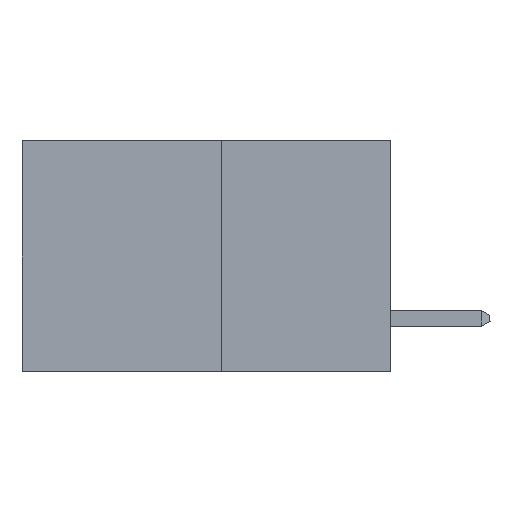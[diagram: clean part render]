
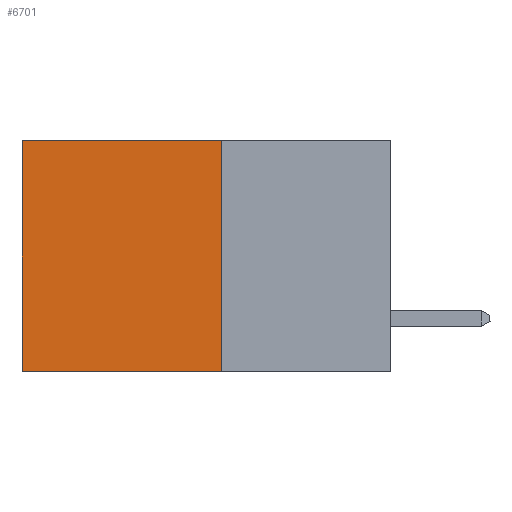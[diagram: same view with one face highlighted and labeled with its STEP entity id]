
A CAD part, left-side view. The second image highlights one B-rep face of the part: STEP entity #6701.
In plain terms, the highlighted planar face has unit normal (-1, 0, 0).
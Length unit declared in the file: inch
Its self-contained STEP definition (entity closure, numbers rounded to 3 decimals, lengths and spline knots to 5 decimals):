
#8 = LINE ( 'NONE', #911, #14515 ) ;
#165 = EDGE_CURVE ( 'NONE', #3886, #6773, #2893, .T. ) ;
#326 = EDGE_CURVE ( 'NONE', #501, #8217, #6914, .T. ) ;
#501 = VERTEX_POINT ( 'NONE', #16231 ) ;
#911 = CARTESIAN_POINT ( 'NONE',  ( 0.277, 0.27, -0.37 ) ) ;
#1520 = DIRECTION ( 'NONE',  ( 1., 0., 0. ) ) ;
#1638 = DIRECTION ( 'NONE',  ( 0., 0., -1. ) ) ;
#2648 = VECTOR ( 'NONE', #5452, 39.37008 ) ;
#2655 = VECTOR ( 'NONE', #4119, 39.37008 ) ;
#2671 = CARTESIAN_POINT ( 'NONE',  ( 0.277, 0.27, -0.37 ) ) ;
#2893 = LINE ( 'NONE', #2671, #5375 ) ;
#3051 = FACE_OUTER_BOUND ( 'NONE', #3517, .T. ) ;
#3517 = EDGE_LOOP ( 'NONE', ( #6762, #16925, #12259, #4838 ) ) ;
#3886 = VERTEX_POINT ( 'NONE', #9211 ) ;
#4119 = DIRECTION ( 'NONE',  ( 0., 0., -1. ) ) ;
#4333 = CARTESIAN_POINT ( 'NONE',  ( 0.277, 0.59, -0.37 ) ) ;
#4524 = CARTESIAN_POINT ( 'NONE',  ( 0.277, 0.27, -0.37 ) ) ;
#4838 = ORIENTED_EDGE ( 'NONE', *, *, #5401, .T. ) ;
#5375 = VECTOR ( 'NONE', #1638, 39.37008 ) ;
#5401 = EDGE_CURVE ( 'NONE', #3886, #501, #9700, .T. ) ;
#5452 = DIRECTION ( 'NONE',  ( 0., 1., 0. ) ) ;
#6701 = ADVANCED_FACE ( 'NONE', ( #3051 ), #16806, .F. ) ;
#6762 = ORIENTED_EDGE ( 'NONE', *, *, #326, .T. ) ;
#6773 = VERTEX_POINT ( 'NONE', #4524 ) ;
#6914 = LINE ( 'NONE', #14420, #2655 ) ;
#8217 = VERTEX_POINT ( 'NONE', #4333 ) ;
#9211 = CARTESIAN_POINT ( 'NONE',  ( 0.277, 0.27, 0. ) ) ;
#9700 = LINE ( 'NONE', #16500, #2648 ) ;
#10567 = EDGE_CURVE ( 'NONE', #6773, #8217, #8, .T. ) ;
#11349 = DIRECTION ( 'NONE',  ( 0., 0., -1. ) ) ;
#12259 = ORIENTED_EDGE ( 'NONE', *, *, #165, .F. ) ;
#13552 = DIRECTION ( 'NONE',  ( 0., 1., 0. ) ) ;
#14021 = AXIS2_PLACEMENT_3D ( 'NONE', #14072, #1520, #11349 ) ;
#14072 = CARTESIAN_POINT ( 'NONE',  ( 0.277, 0.27, -0.37 ) ) ;
#14420 = CARTESIAN_POINT ( 'NONE',  ( 0.277, 0.59, -0.37 ) ) ;
#14515 = VECTOR ( 'NONE', #13552, 39.37008 ) ;
#16231 = CARTESIAN_POINT ( 'NONE',  ( 0.277, 0.59, 0. ) ) ;
#16500 = CARTESIAN_POINT ( 'NONE',  ( 0.277, 0.27, 0. ) ) ;
#16806 = PLANE ( 'NONE',  #14021 ) ;
#16925 = ORIENTED_EDGE ( 'NONE', *, *, #10567, .F. ) ;
